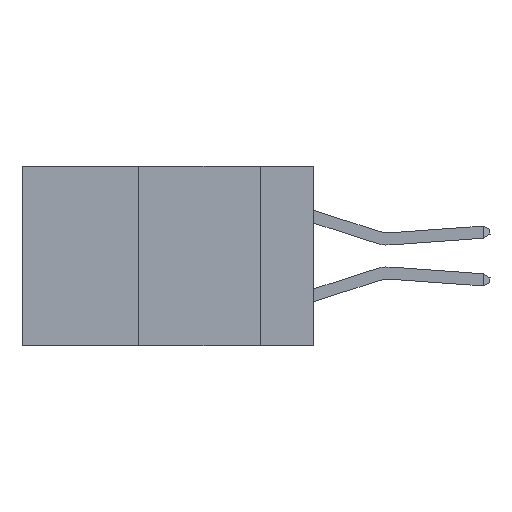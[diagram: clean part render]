
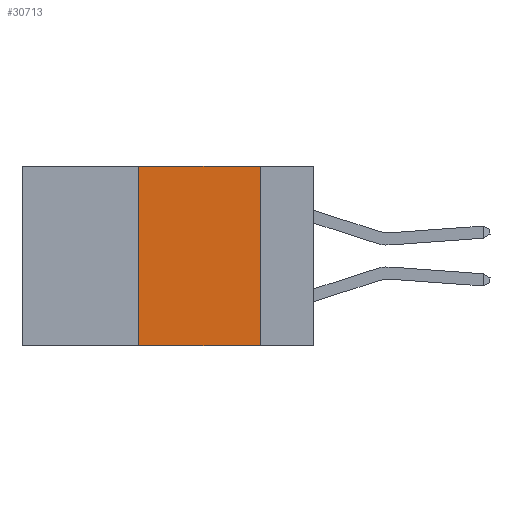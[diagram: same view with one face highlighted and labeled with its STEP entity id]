
A CAD part, left-side view. The second image highlights one B-rep face of the part: STEP entity #30713.
In plain terms, the highlighted planar face has unit normal (-1, 0, 0).
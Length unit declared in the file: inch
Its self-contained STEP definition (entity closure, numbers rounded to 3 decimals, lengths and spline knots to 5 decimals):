
#216 = FACE_OUTER_BOUND ( 'NONE', #23582, .T. ) ;
#1436 = CARTESIAN_POINT ( 'NONE',  ( 0., 0.11, -0.37 ) ) ;
#1619 = VERTEX_POINT ( 'NONE', #1436 ) ;
#3022 = EDGE_CURVE ( 'NONE', #24009, #1619, #10079, .T. ) ;
#3232 = DIRECTION ( 'NONE',  ( 0., -1., 0. ) ) ;
#4879 = EDGE_CURVE ( 'NONE', #24009, #13637, #8412, .T. ) ;
#5131 = CARTESIAN_POINT ( 'NONE',  ( 0., 0.6, 0. ) ) ;
#5752 = CARTESIAN_POINT ( 'NONE',  ( 0., 0.36, -0.37 ) ) ;
#6311 = EDGE_CURVE ( 'NONE', #13637, #11842, #30690, .T. ) ;
#7314 = CARTESIAN_POINT ( 'NONE',  ( 0., 0.11, 0. ) ) ;
#7885 = AXIS2_PLACEMENT_3D ( 'NONE', #5131, #10077, #20127 ) ;
#8311 = CARTESIAN_POINT ( 'NONE',  ( 0., 0.6, -0.37 ) ) ;
#8412 = LINE ( 'NONE', #14248, #10701 ) ;
#9105 = VECTOR ( 'NONE', #26005, 39.37008 ) ;
#10077 = DIRECTION ( 'NONE',  ( 1., 0., 0. ) ) ;
#10079 = LINE ( 'NONE', #8311, #15899 ) ;
#10701 = VECTOR ( 'NONE', #31481, 39.37008 ) ;
#11842 = VERTEX_POINT ( 'NONE', #15275 ) ;
#13637 = VERTEX_POINT ( 'NONE', #18230 ) ;
#13797 = ORIENTED_EDGE ( 'NONE', *, *, #3022, .T. ) ;
#14020 = ORIENTED_EDGE ( 'NONE', *, *, #6311, .F. ) ;
#14248 = CARTESIAN_POINT ( 'NONE',  ( 0., 0.36, 0. ) ) ;
#15275 = CARTESIAN_POINT ( 'NONE',  ( 0., 0.11, 0. ) ) ;
#15899 = VECTOR ( 'NONE', #3232, 39.37008 ) ;
#18230 = CARTESIAN_POINT ( 'NONE',  ( 0., 0.36, 0. ) ) ;
#18572 = CARTESIAN_POINT ( 'NONE',  ( 0., 0.6, 0. ) ) ;
#20127 = DIRECTION ( 'NONE',  ( 0., 0., -1. ) ) ;
#22282 = PLANE ( 'NONE',  #7885 ) ;
#22589 = EDGE_CURVE ( 'NONE', #11842, #1619, #29958, .T. ) ;
#22632 = VECTOR ( 'NONE', #26959, 39.37008 ) ;
#22884 = ORIENTED_EDGE ( 'NONE', *, *, #22589, .F. ) ;
#23582 = EDGE_LOOP ( 'NONE', ( #22884, #14020, #26947, #13797 ) ) ;
#24009 = VERTEX_POINT ( 'NONE', #5752 ) ;
#26005 = DIRECTION ( 'NONE',  ( 0., -1., 0. ) ) ;
#26947 = ORIENTED_EDGE ( 'NONE', *, *, #4879, .F. ) ;
#26959 = DIRECTION ( 'NONE',  ( 0., 0., -1. ) ) ;
#29958 = LINE ( 'NONE', #7314, #22632 ) ;
#30690 = LINE ( 'NONE', #18572, #9105 ) ;
#30713 = ADVANCED_FACE ( 'NONE', ( #216 ), #22282, .F. ) ;
#31481 = DIRECTION ( 'NONE',  ( 0., 0., 1. ) ) ;
